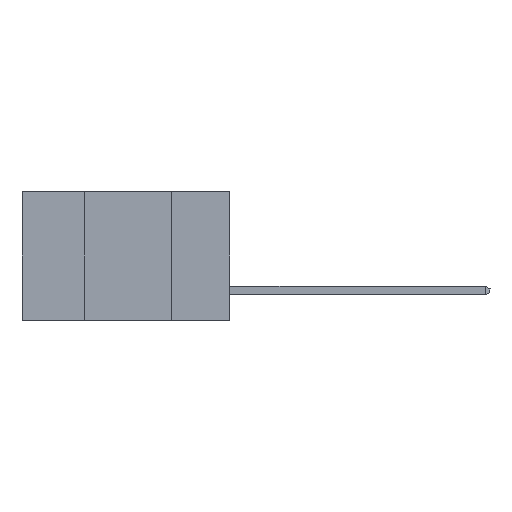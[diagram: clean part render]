
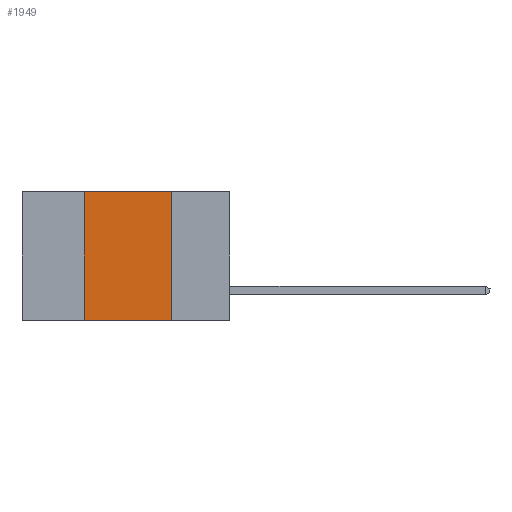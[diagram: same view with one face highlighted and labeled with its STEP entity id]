
A CAD part, left-side view. The second image highlights one B-rep face of the part: STEP entity #1949.
In plain terms, the highlighted planar face has unit normal (-1, 0, 0).
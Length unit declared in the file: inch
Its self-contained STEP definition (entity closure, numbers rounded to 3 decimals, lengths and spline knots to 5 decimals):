
#349 = DIRECTION ( 'NONE',  ( 0., -1., 0. ) ) ;
#721 = CARTESIAN_POINT ( 'NONE',  ( 0., 0.6, 0. ) ) ;
#858 = EDGE_LOOP ( 'NONE', ( #6026, #5908, #3660, #12331 ) ) ;
#1385 = CARTESIAN_POINT ( 'NONE',  ( 0., 0.17, 0. ) ) ;
#1404 = LINE ( 'NONE', #2598, #13956 ) ;
#1537 = LINE ( 'NONE', #3597, #3537 ) ;
#1949 = ADVANCED_FACE ( 'NONE', ( #5432 ), #14416, .F. ) ;
#2535 = VERTEX_POINT ( 'NONE', #6220 ) ;
#2598 = CARTESIAN_POINT ( 'NONE',  ( 0., 0.42, -0.37 ) ) ;
#3537 = VECTOR ( 'NONE', #349, 39.37008 ) ;
#3557 = EDGE_CURVE ( 'NONE', #10411, #2535, #1404, .T. ) ;
#3597 = CARTESIAN_POINT ( 'NONE',  ( 0., 0.6, -0.37 ) ) ;
#3660 = ORIENTED_EDGE ( 'NONE', *, *, #3557, .F. ) ;
#4553 = CARTESIAN_POINT ( 'NONE',  ( 0., 0.42, -0.37 ) ) ;
#4605 = CARTESIAN_POINT ( 'NONE',  ( 0., 0.17, -0.37 ) ) ;
#5226 = DIRECTION ( 'NONE',  ( 0., -1., 0. ) ) ;
#5432 = FACE_OUTER_BOUND ( 'NONE', #858, .T. ) ;
#5908 = ORIENTED_EDGE ( 'NONE', *, *, #13846, .F. ) ;
#6026 = ORIENTED_EDGE ( 'NONE', *, *, #10550, .F. ) ;
#6220 = CARTESIAN_POINT ( 'NONE',  ( 0., 0.42, 0. ) ) ;
#6902 = DIRECTION ( 'NONE',  ( 0., 0., -1. ) ) ;
#7071 = DIRECTION ( 'NONE',  ( 0., 0., 1. ) ) ;
#7492 = CARTESIAN_POINT ( 'NONE',  ( 0., 0.6, 0. ) ) ;
#8956 = LINE ( 'NONE', #13464, #10750 ) ;
#9124 = VERTEX_POINT ( 'NONE', #4605 ) ;
#10273 = DIRECTION ( 'NONE',  ( 0., 0., -1. ) ) ;
#10411 = VERTEX_POINT ( 'NONE', #4553 ) ;
#10550 = EDGE_CURVE ( 'NONE', #14031, #9124, #8956, .T. ) ;
#10750 = VECTOR ( 'NONE', #10273, 39.37008 ) ;
#10793 = LINE ( 'NONE', #721, #12221 ) ;
#11958 = DIRECTION ( 'NONE',  ( 1., 0., 0. ) ) ;
#12221 = VECTOR ( 'NONE', #5226, 39.37008 ) ;
#12331 = ORIENTED_EDGE ( 'NONE', *, *, #12929, .T. ) ;
#12929 = EDGE_CURVE ( 'NONE', #10411, #9124, #1537, .T. ) ;
#13464 = CARTESIAN_POINT ( 'NONE',  ( 0., 0.17, -0.37 ) ) ;
#13846 = EDGE_CURVE ( 'NONE', #2535, #14031, #10793, .T. ) ;
#13956 = VECTOR ( 'NONE', #7071, 39.37008 ) ;
#14031 = VERTEX_POINT ( 'NONE', #1385 ) ;
#14154 = AXIS2_PLACEMENT_3D ( 'NONE', #7492, #11958, #6902 ) ;
#14416 = PLANE ( 'NONE',  #14154 ) ;
